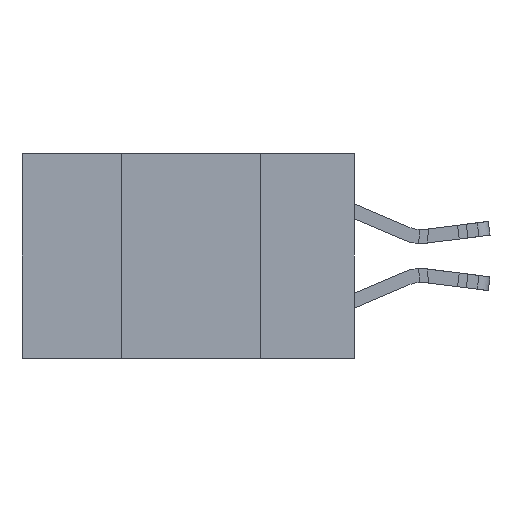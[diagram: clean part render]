
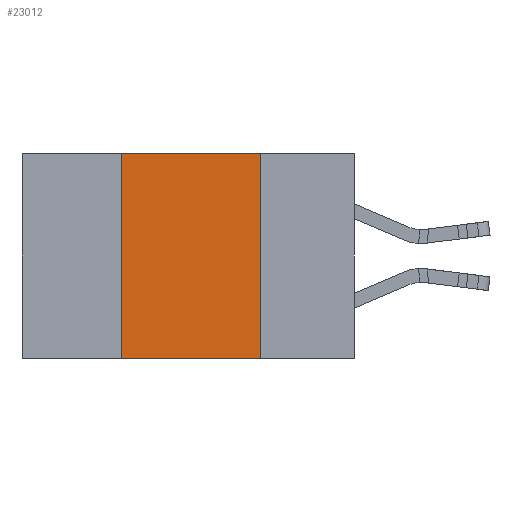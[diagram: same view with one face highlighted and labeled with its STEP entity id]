
A CAD part, left-side view. The second image highlights one B-rep face of the part: STEP entity #23012.
In plain terms, the highlighted planar face has unit normal (-1, 0, 0).
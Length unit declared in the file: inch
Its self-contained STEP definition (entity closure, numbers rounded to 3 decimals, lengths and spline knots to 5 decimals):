
#266 = EDGE_CURVE ( 'NONE', #20039, #5227, #13864, .T. ) ;
#2077 = VERTEX_POINT ( 'NONE', #8337 ) ;
#2387 = VECTOR ( 'NONE', #10654, 39.37008 ) ;
#2881 = CARTESIAN_POINT ( 'NONE',  ( 0., 0.42, -0.37 ) ) ;
#3317 = EDGE_LOOP ( 'NONE', ( #20494, #11901, #5878, #19889 ) ) ;
#3569 = AXIS2_PLACEMENT_3D ( 'NONE', #8378, #16500, #8902 ) ;
#5227 = VERTEX_POINT ( 'NONE', #10948 ) ;
#5878 = ORIENTED_EDGE ( 'NONE', *, *, #13012, .F. ) ;
#6163 = VECTOR ( 'NONE', #8999, 39.37008 ) ;
#7487 = VECTOR ( 'NONE', #20253, 39.37008 ) ;
#8124 = DIRECTION ( 'NONE',  ( 0., -1., 0. ) ) ;
#8337 = CARTESIAN_POINT ( 'NONE',  ( 0., 0.17, 0. ) ) ;
#8345 = VECTOR ( 'NONE', #8124, 39.37008 ) ;
#8378 = CARTESIAN_POINT ( 'NONE',  ( 0., 0.6, 0. ) ) ;
#8902 = DIRECTION ( 'NONE',  ( 0., 0., -1. ) ) ;
#8999 = DIRECTION ( 'NONE',  ( 0., 0., -1. ) ) ;
#10654 = DIRECTION ( 'NONE',  ( 0., 0., 1. ) ) ;
#10679 = PLANE ( 'NONE',  #3569 ) ;
#10948 = CARTESIAN_POINT ( 'NONE',  ( 0., 0.17, -0.37 ) ) ;
#10969 = CARTESIAN_POINT ( 'NONE',  ( 0., 0.42, 0. ) ) ;
#11901 = ORIENTED_EDGE ( 'NONE', *, *, #19446, .F. ) ;
#12819 = LINE ( 'NONE', #2881, #2387 ) ;
#13012 = EDGE_CURVE ( 'NONE', #20039, #22567, #12819, .T. ) ;
#13864 = LINE ( 'NONE', #21590, #8345 ) ;
#14261 = EDGE_CURVE ( 'NONE', #2077, #5227, #18647, .T. ) ;
#14844 = CARTESIAN_POINT ( 'NONE',  ( 0., 0.17, -0.37 ) ) ;
#16500 = DIRECTION ( 'NONE',  ( 1., 0., 0. ) ) ;
#18647 = LINE ( 'NONE', #14844, #6163 ) ;
#18722 = CARTESIAN_POINT ( 'NONE',  ( 0., 0.6, 0. ) ) ;
#19446 = EDGE_CURVE ( 'NONE', #22567, #2077, #22399, .T. ) ;
#19889 = ORIENTED_EDGE ( 'NONE', *, *, #266, .T. ) ;
#20039 = VERTEX_POINT ( 'NONE', #23905 ) ;
#20253 = DIRECTION ( 'NONE',  ( 0., -1., 0. ) ) ;
#20494 = ORIENTED_EDGE ( 'NONE', *, *, #14261, .F. ) ;
#21590 = CARTESIAN_POINT ( 'NONE',  ( 0., 0.6, -0.37 ) ) ;
#22399 = LINE ( 'NONE', #18722, #7487 ) ;
#22567 = VERTEX_POINT ( 'NONE', #10969 ) ;
#23012 = ADVANCED_FACE ( 'NONE', ( #24374 ), #10679, .F. ) ;
#23905 = CARTESIAN_POINT ( 'NONE',  ( 0., 0.42, -0.37 ) ) ;
#24374 = FACE_OUTER_BOUND ( 'NONE', #3317, .T. ) ;
